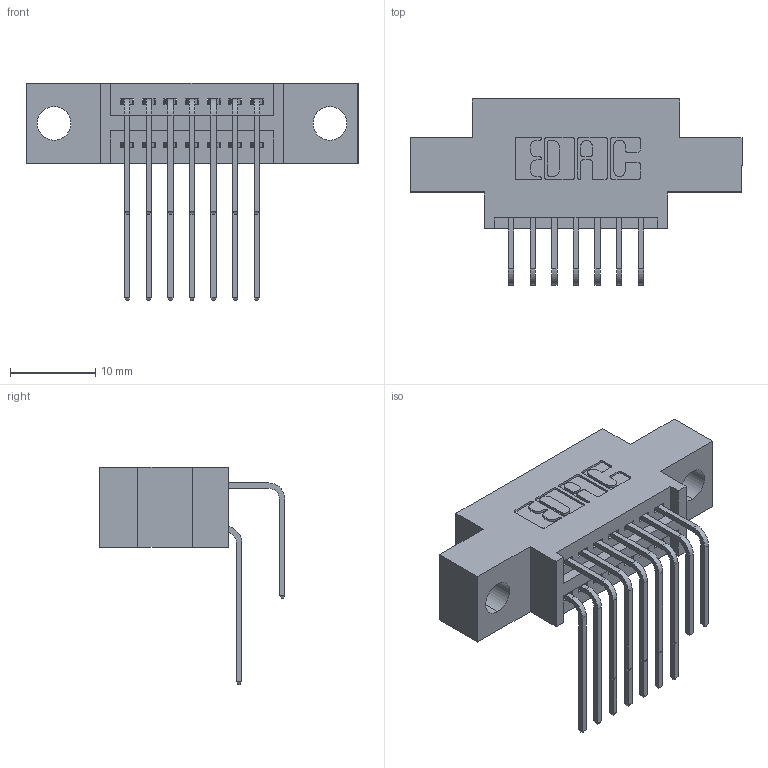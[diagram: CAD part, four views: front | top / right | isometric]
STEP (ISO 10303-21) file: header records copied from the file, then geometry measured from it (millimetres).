
FILE_DESCRIPTION (( 'STEP AP203' ), '1' );
FILE_NAME ('345-014-558-804.STEP', '2021-05-19T16:08:48', ( '' ), ( '' ), 'SwSTEP 2.0', 'SolidWorks 2020', '' );
FILE_SCHEMA (( 'CONFIG_CONTROL_DESIGN' ));
Length unit declared in the file: inch
Products named in the file (4): 345 Part_0.170 Offset - 0.156 Dia-TI; 345-292-001_558 559 Tail - 1; 345-292-001_558 Tail - 2; 345-014-558-804
Assembly tree (15 placements, depth 2):
  345-014-558-804
    345 Part_0.170 Offset - 0.156 Dia-TI
    345-292-001_558 559 Tail - 1  x7
    345-292-001_558 Tail - 2  x7
Bounding box: 38.99 x 21.83 x 25.53 mm (x, y, z)
Volume: 3324 mm3; surface area: 4610.4 mm2
Topology: 15 solids, 15 shells, 872 faces, 2559 edges, 1686 vertices
Faces by surface type: plane 588, cylinder 284
Entity records: 12407 total; most frequent: CARTESIAN_POINT 2165, ORIENTED_EDGE 2046, DIRECTION 1923, EDGE_CURVE 1023, VECTOR 823, LINE 823, VERTEX_POINT 678, AXIS2_PLACEMENT_3D 550
